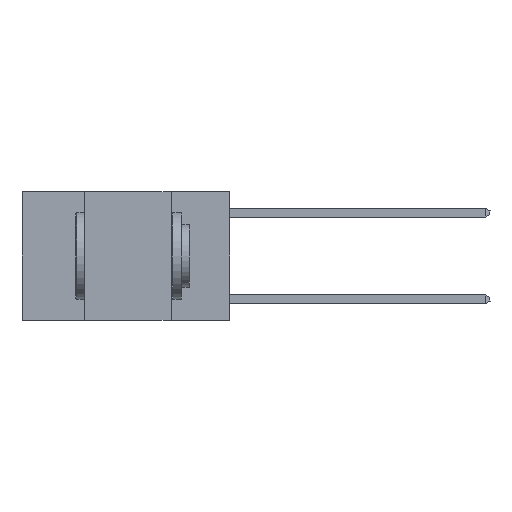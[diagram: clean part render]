
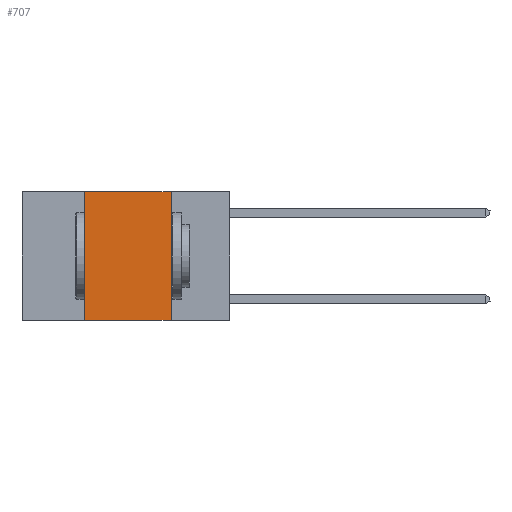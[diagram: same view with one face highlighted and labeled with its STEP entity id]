
A CAD part, left-side view. The second image highlights one B-rep face of the part: STEP entity #707.
In plain terms, the highlighted planar face has unit normal (-1, 0, 0).
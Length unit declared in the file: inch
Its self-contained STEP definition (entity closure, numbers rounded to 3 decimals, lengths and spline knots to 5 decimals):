
#534 = CARTESIAN_POINT ( 'NONE',  ( 0., 0.6, 0. ) ) ;
#567 = EDGE_LOOP ( 'NONE', ( #4865, #1952, #12240, #1233 ) ) ;
#707 = ADVANCED_FACE ( 'NONE', ( #4000 ), #11718, .F. ) ;
#737 = EDGE_CURVE ( 'NONE', #9265, #3993, #12731, .T. ) ;
#1233 = ORIENTED_EDGE ( 'NONE', *, *, #9860, .T. ) ;
#1472 = EDGE_CURVE ( 'NONE', #4240, #9265, #5988, .T. ) ;
#1904 = LINE ( 'NONE', #3281, #8820 ) ;
#1909 = DIRECTION ( 'NONE',  ( 1., 0., 0. ) ) ;
#1952 = ORIENTED_EDGE ( 'NONE', *, *, #1472, .F. ) ;
#2118 = VECTOR ( 'NONE', #2996, 39.37008 ) ;
#2142 = VECTOR ( 'NONE', #9973, 39.37008 ) ;
#2996 = DIRECTION ( 'NONE',  ( 0., 0., -1. ) ) ;
#3147 = CARTESIAN_POINT ( 'NONE',  ( 0., 0.6, 0. ) ) ;
#3206 = CARTESIAN_POINT ( 'NONE',  ( 0., 0.42, -0.37 ) ) ;
#3281 = CARTESIAN_POINT ( 'NONE',  ( 0., 0.42, 0. ) ) ;
#3919 = DIRECTION ( 'NONE',  ( 0., 0., -1. ) ) ;
#3993 = VERTEX_POINT ( 'NONE', #8914 ) ;
#4000 = FACE_OUTER_BOUND ( 'NONE', #567, .T. ) ;
#4028 = CARTESIAN_POINT ( 'NONE',  ( 0., 0.42, 0. ) ) ;
#4240 = VERTEX_POINT ( 'NONE', #4028 ) ;
#4826 = LINE ( 'NONE', #10301, #2142 ) ;
#4865 = ORIENTED_EDGE ( 'NONE', *, *, #737, .F. ) ;
#4883 = DIRECTION ( 'NONE',  ( 0., -1., 0. ) ) ;
#5113 = VECTOR ( 'NONE', #4883, 39.37008 ) ;
#5201 = DIRECTION ( 'NONE',  ( 0., 0., 1. ) ) ;
#5988 = LINE ( 'NONE', #534, #5113 ) ;
#8820 = VECTOR ( 'NONE', #5201, 39.37008 ) ;
#8914 = CARTESIAN_POINT ( 'NONE',  ( 0., 0.17, -0.37 ) ) ;
#9265 = VERTEX_POINT ( 'NONE', #11131 ) ;
#9462 = AXIS2_PLACEMENT_3D ( 'NONE', #3147, #1909, #3919 ) ;
#9860 = EDGE_CURVE ( 'NONE', #10071, #3993, #4826, .T. ) ;
#9973 = DIRECTION ( 'NONE',  ( 0., -1., 0. ) ) ;
#10071 = VERTEX_POINT ( 'NONE', #3206 ) ;
#10301 = CARTESIAN_POINT ( 'NONE',  ( 0., 0.6, -0.37 ) ) ;
#11131 = CARTESIAN_POINT ( 'NONE',  ( 0., 0.17, 0. ) ) ;
#11718 = PLANE ( 'NONE',  #9462 ) ;
#12240 = ORIENTED_EDGE ( 'NONE', *, *, #13195, .F. ) ;
#12731 = LINE ( 'NONE', #14016, #2118 ) ;
#13195 = EDGE_CURVE ( 'NONE', #10071, #4240, #1904, .T. ) ;
#14016 = CARTESIAN_POINT ( 'NONE',  ( 0., 0.17, 0. ) ) ;
